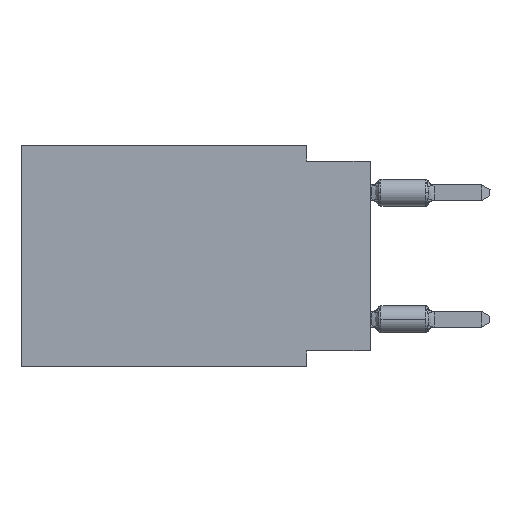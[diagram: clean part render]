
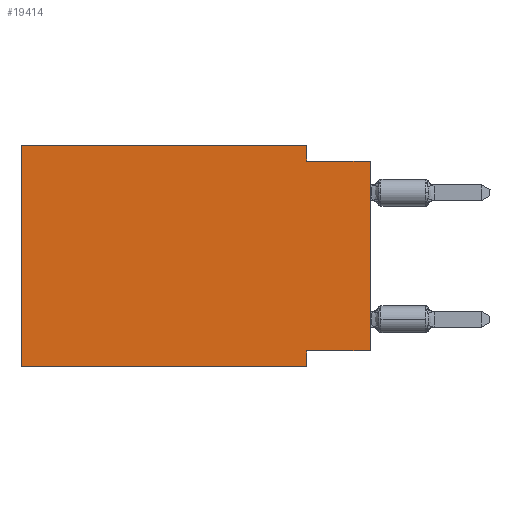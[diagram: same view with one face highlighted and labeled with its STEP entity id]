
A CAD part, left-side view. The second image highlights one B-rep face of the part: STEP entity #19414.
In plain terms, the highlighted planar face has unit normal (-1, 0, 0).
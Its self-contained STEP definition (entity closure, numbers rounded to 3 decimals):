
#604 = DIRECTION ( 'NONE',  ( 0., 1., 0. ) ) ;
#1474 = LINE ( 'NONE', #18671, #3347 ) ;
#2790 = LINE ( 'NONE', #14308, #34306 ) ;
#3029 = LINE ( 'NONE', #29053, #6972 ) ;
#3320 = ORIENTED_EDGE ( 'NONE', *, *, #5862, .F. ) ;
#3347 = VECTOR ( 'NONE', #29768, 1000. ) ;
#4183 = CARTESIAN_POINT ( 'NONE',  ( 0., 13.97, 0. ) ) ;
#4543 = DIRECTION ( 'NONE',  ( 0., 0., -1. ) ) ;
#4906 = LINE ( 'NONE', #11321, #17806 ) ;
#5274 = EDGE_CURVE ( 'NONE', #17406, #23241, #4906, .T. ) ;
#5502 = EDGE_CURVE ( 'NONE', #36473, #24771, #1474, .T. ) ;
#5846 = VERTEX_POINT ( 'NONE', #28799 ) ;
#5862 = EDGE_CURVE ( 'NONE', #17406, #36473, #28421, .T. ) ;
#6221 = VECTOR ( 'NONE', #20198, 1000. ) ;
#6972 = VECTOR ( 'NONE', #28675, 1000. ) ;
#8137 = CARTESIAN_POINT ( 'NONE',  ( 0., 2.54, 0. ) ) ;
#8504 = EDGE_CURVE ( 'NONE', #24771, #35161, #8693, .T. ) ;
#8693 = LINE ( 'NONE', #8137, #6221 ) ;
#8701 = EDGE_CURVE ( 'NONE', #5846, #32015, #24517, .T. ) ;
#9596 = ORIENTED_EDGE ( 'NONE', *, *, #8701, .T. ) ;
#11241 = EDGE_CURVE ( 'NONE', #35161, #32015, #2790, .T. ) ;
#11321 = CARTESIAN_POINT ( 'NONE',  ( 0., 13.97, -8.89 ) ) ;
#12880 = VECTOR ( 'NONE', #30173, 1000. ) ;
#14308 = CARTESIAN_POINT ( 'NONE',  ( 0., 0., -0.635 ) ) ;
#14523 = CARTESIAN_POINT ( 'NONE',  ( 0., 13.97, -8.89 ) ) ;
#15444 = ORIENTED_EDGE ( 'NONE', *, *, #21586, .F. ) ;
#17013 = CARTESIAN_POINT ( 'NONE',  ( 0., 2.54, 0. ) ) ;
#17117 = CARTESIAN_POINT ( 'NONE',  ( 0., 13.97, 0. ) ) ;
#17224 = ORIENTED_EDGE ( 'NONE', *, *, #5274, .T. ) ;
#17300 = DIRECTION ( 'NONE',  ( 0., 0., 1. ) ) ;
#17406 = VERTEX_POINT ( 'NONE', #14523 ) ;
#17747 = VECTOR ( 'NONE', #17300, 1000. ) ;
#17806 = VECTOR ( 'NONE', #25445, 1000. ) ;
#18004 = CARTESIAN_POINT ( 'NONE',  ( 0., 0., -0.635 ) ) ;
#18106 = ORIENTED_EDGE ( 'NONE', *, *, #5502, .F. ) ;
#18127 = EDGE_LOOP ( 'NONE', ( #9596, #28396, #35737, #18106, #3320, #17224, #15444, #30631 ) ) ;
#18671 = CARTESIAN_POINT ( 'NONE',  ( 0., 13.97, 0. ) ) ;
#19414 = ADVANCED_FACE ( 'NONE', ( #24179 ), #33035, .F. ) ;
#20198 = DIRECTION ( 'NONE',  ( 0., 0., -1. ) ) ;
#20784 = CARTESIAN_POINT ( 'NONE',  ( 0., 0., -8.255 ) ) ;
#21586 = EDGE_CURVE ( 'NONE', #25341, #23241, #3029, .T. ) ;
#23241 = VERTEX_POINT ( 'NONE', #27535 ) ;
#24177 = LINE ( 'NONE', #20784, #29168 ) ;
#24179 = FACE_OUTER_BOUND ( 'NONE', #18127, .T. ) ;
#24517 = LINE ( 'NONE', #33189, #12880 ) ;
#24771 = VERTEX_POINT ( 'NONE', #17013 ) ;
#25012 = AXIS2_PLACEMENT_3D ( 'NONE', #4183, #33213, #4543 ) ;
#25341 = VERTEX_POINT ( 'NONE', #27263 ) ;
#25445 = DIRECTION ( 'NONE',  ( 0., -1., 0. ) ) ;
#25606 = DIRECTION ( 'NONE',  ( 0., -1., 0. ) ) ;
#27263 = CARTESIAN_POINT ( 'NONE',  ( 0., 2.54, -8.255 ) ) ;
#27535 = CARTESIAN_POINT ( 'NONE',  ( 0., 2.54, -8.89 ) ) ;
#28396 = ORIENTED_EDGE ( 'NONE', *, *, #11241, .F. ) ;
#28421 = LINE ( 'NONE', #17117, #17747 ) ;
#28675 = DIRECTION ( 'NONE',  ( 0., 0., -1. ) ) ;
#28799 = CARTESIAN_POINT ( 'NONE',  ( 0., 0., -8.255 ) ) ;
#29053 = CARTESIAN_POINT ( 'NONE',  ( 0., 2.54, -8.89 ) ) ;
#29168 = VECTOR ( 'NONE', #604, 1000. ) ;
#29768 = DIRECTION ( 'NONE',  ( 0., -1., 0. ) ) ;
#30173 = DIRECTION ( 'NONE',  ( 0., 0., 1. ) ) ;
#30631 = ORIENTED_EDGE ( 'NONE', *, *, #32440, .F. ) ;
#32015 = VERTEX_POINT ( 'NONE', #18004 ) ;
#32440 = EDGE_CURVE ( 'NONE', #5846, #25341, #24177, .T. ) ;
#33035 = PLANE ( 'NONE',  #25012 ) ;
#33189 = CARTESIAN_POINT ( 'NONE',  ( 0., 0., 0. ) ) ;
#33213 = DIRECTION ( 'NONE',  ( 1., 0., 0. ) ) ;
#34306 = VECTOR ( 'NONE', #25606, 1000. ) ;
#35161 = VERTEX_POINT ( 'NONE', #35942 ) ;
#35737 = ORIENTED_EDGE ( 'NONE', *, *, #8504, .F. ) ;
#35942 = CARTESIAN_POINT ( 'NONE',  ( 0., 2.54, -0.635 ) ) ;
#36308 = CARTESIAN_POINT ( 'NONE',  ( 0., 13.97, 0. ) ) ;
#36473 = VERTEX_POINT ( 'NONE', #36308 ) ;
